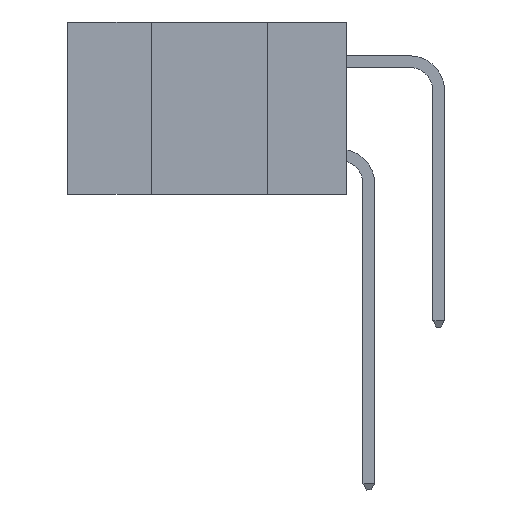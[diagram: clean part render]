
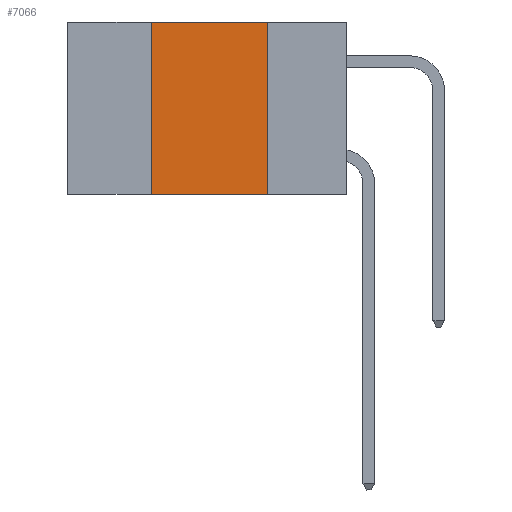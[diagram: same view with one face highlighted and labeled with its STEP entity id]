
A CAD part, left-side view. The second image highlights one B-rep face of the part: STEP entity #7066.
In plain terms, the highlighted planar face has unit normal (-1, 0, 0).
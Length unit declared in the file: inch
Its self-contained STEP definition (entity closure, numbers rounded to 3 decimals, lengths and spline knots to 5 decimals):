
#857 = EDGE_CURVE ( 'NONE', #13701, #7667, #16942, .T. ) ;
#861 = ORIENTED_EDGE ( 'NONE', *, *, #7379, .F. ) ;
#923 = CARTESIAN_POINT ( 'NONE',  ( 0., 0.42, -0.37 ) ) ;
#2007 = DIRECTION ( 'NONE',  ( 0., 0., 1. ) ) ;
#2399 = AXIS2_PLACEMENT_3D ( 'NONE', #17100, #4778, #14421 ) ;
#2448 = EDGE_LOOP ( 'NONE', ( #15993, #12354, #861, #7832 ) ) ;
#2848 = CARTESIAN_POINT ( 'NONE',  ( 0., 0.6, 0. ) ) ;
#3332 = VERTEX_POINT ( 'NONE', #9259 ) ;
#4292 = DIRECTION ( 'NONE',  ( 0., -1., 0. ) ) ;
#4521 = VECTOR ( 'NONE', #4292, 39.37008 ) ;
#4778 = DIRECTION ( 'NONE',  ( 1., 0., 0. ) ) ;
#5282 = VERTEX_POINT ( 'NONE', #923 ) ;
#6780 = CARTESIAN_POINT ( 'NONE',  ( 0., 0.17, -0.37 ) ) ;
#7066 = ADVANCED_FACE ( 'NONE', ( #8441 ), #13041, .F. ) ;
#7379 = EDGE_CURVE ( 'NONE', #5282, #3332, #16590, .T. ) ;
#7667 = VERTEX_POINT ( 'NONE', #6780 ) ;
#7832 = ORIENTED_EDGE ( 'NONE', *, *, #12024, .T. ) ;
#8208 = LINE ( 'NONE', #11220, #4521 ) ;
#8238 = CARTESIAN_POINT ( 'NONE',  ( 0., 0.17, 0. ) ) ;
#8366 = CARTESIAN_POINT ( 'NONE',  ( 0., 0.17, 0. ) ) ;
#8441 = FACE_OUTER_BOUND ( 'NONE', #2448, .T. ) ;
#9259 = CARTESIAN_POINT ( 'NONE',  ( 0., 0.42, 0. ) ) ;
#9592 = LINE ( 'NONE', #2848, #12810 ) ;
#9665 = VECTOR ( 'NONE', #10408, 39.37008 ) ;
#10230 = EDGE_CURVE ( 'NONE', #3332, #13701, #9592, .T. ) ;
#10408 = DIRECTION ( 'NONE',  ( 0., 0., -1. ) ) ;
#11220 = CARTESIAN_POINT ( 'NONE',  ( 0., 0.6, -0.37 ) ) ;
#12024 = EDGE_CURVE ( 'NONE', #5282, #7667, #8208, .T. ) ;
#12354 = ORIENTED_EDGE ( 'NONE', *, *, #10230, .F. ) ;
#12810 = VECTOR ( 'NONE', #13883, 39.37008 ) ;
#12963 = VECTOR ( 'NONE', #2007, 39.37008 ) ;
#13041 = PLANE ( 'NONE',  #2399 ) ;
#13701 = VERTEX_POINT ( 'NONE', #8366 ) ;
#13883 = DIRECTION ( 'NONE',  ( 0., -1., 0. ) ) ;
#14421 = DIRECTION ( 'NONE',  ( 0., 0., -1. ) ) ;
#15751 = CARTESIAN_POINT ( 'NONE',  ( 0., 0.42, 0. ) ) ;
#15993 = ORIENTED_EDGE ( 'NONE', *, *, #857, .F. ) ;
#16590 = LINE ( 'NONE', #15751, #12963 ) ;
#16942 = LINE ( 'NONE', #8238, #9665 ) ;
#17100 = CARTESIAN_POINT ( 'NONE',  ( 0., 0.6, 0. ) ) ;
